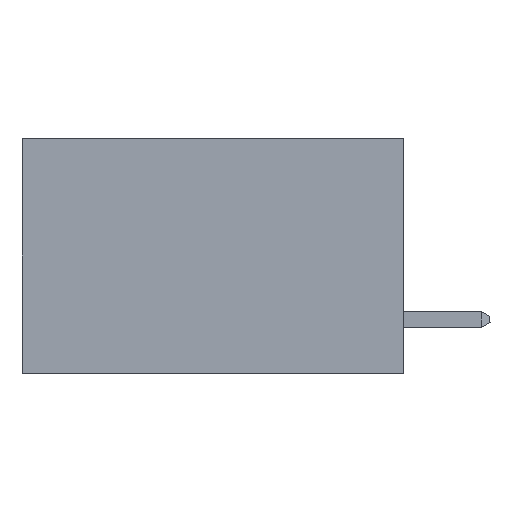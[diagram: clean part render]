
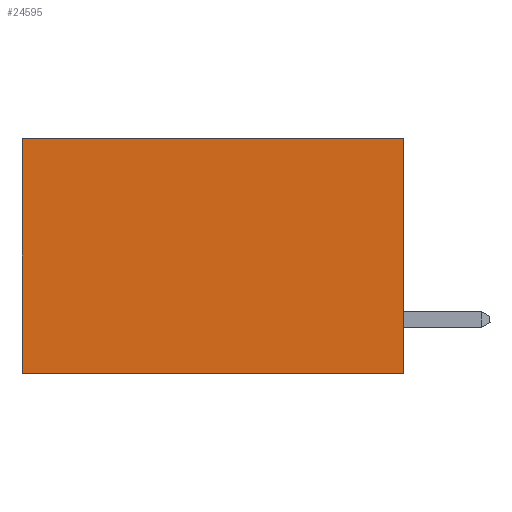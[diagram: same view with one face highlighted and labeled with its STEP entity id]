
A CAD part, left-side view. The second image highlights one B-rep face of the part: STEP entity #24595.
In plain terms, the highlighted planar face has unit normal (-1, 0, 0).
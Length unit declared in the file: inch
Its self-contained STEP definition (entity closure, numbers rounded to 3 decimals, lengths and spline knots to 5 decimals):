
#133 = ORIENTED_EDGE ( 'NONE', *, *, #6053, .F. ) ;
#842 = CARTESIAN_POINT ( 'NONE',  ( 0.2875, 0.6, 0. ) ) ;
#1766 = EDGE_LOOP ( 'NONE', ( #18951, #10182, #133, #32481 ) ) ;
#2347 = AXIS2_PLACEMENT_3D ( 'NONE', #10885, #22368, #5000 ) ;
#3352 = LINE ( 'NONE', #7746, #18024 ) ;
#3517 = CARTESIAN_POINT ( 'NONE',  ( 0.2875, 0., 0. ) ) ;
#3577 = CARTESIAN_POINT ( 'NONE',  ( 0.2875, 0., -0.37 ) ) ;
#5000 = DIRECTION ( 'NONE',  ( 0., 0., -1. ) ) ;
#6053 = EDGE_CURVE ( 'NONE', #13426, #7512, #34824, .T. ) ;
#7512 = VERTEX_POINT ( 'NONE', #3577 ) ;
#7746 = CARTESIAN_POINT ( 'NONE',  ( 0.2875, 0., -0.37 ) ) ;
#8296 = CARTESIAN_POINT ( 'NONE',  ( 0.2875, 0., 0. ) ) ;
#8303 = EDGE_CURVE ( 'NONE', #13763, #11509, #19114, .T. ) ;
#8940 = CARTESIAN_POINT ( 'NONE',  ( 0.2875, 0.6, 0. ) ) ;
#9580 = DIRECTION ( 'NONE',  ( 0., 1., 0. ) ) ;
#10182 = ORIENTED_EDGE ( 'NONE', *, *, #18704, .F. ) ;
#10715 = DIRECTION ( 'NONE',  ( 0., 1., 0. ) ) ;
#10885 = CARTESIAN_POINT ( 'NONE',  ( 0.2875, 0., 0. ) ) ;
#11509 = VERTEX_POINT ( 'NONE', #13775 ) ;
#11645 = CARTESIAN_POINT ( 'NONE',  ( 0.2875, 0., 0. ) ) ;
#13426 = VERTEX_POINT ( 'NONE', #8296 ) ;
#13701 = EDGE_CURVE ( 'NONE', #13426, #13763, #28939, .T. ) ;
#13763 = VERTEX_POINT ( 'NONE', #842 ) ;
#13775 = CARTESIAN_POINT ( 'NONE',  ( 0.2875, 0.6, -0.37 ) ) ;
#18024 = VECTOR ( 'NONE', #10715, 39.37008 ) ;
#18704 = EDGE_CURVE ( 'NONE', #7512, #11509, #3352, .T. ) ;
#18951 = ORIENTED_EDGE ( 'NONE', *, *, #8303, .T. ) ;
#19114 = LINE ( 'NONE', #8940, #25795 ) ;
#19523 = PLANE ( 'NONE',  #2347 ) ;
#19675 = VECTOR ( 'NONE', #37185, 39.37008 ) ;
#22368 = DIRECTION ( 'NONE',  ( 1., 0., 0. ) ) ;
#24595 = ADVANCED_FACE ( 'NONE', ( #29223 ), #19523, .F. ) ;
#25795 = VECTOR ( 'NONE', #31814, 39.37008 ) ;
#28049 = VECTOR ( 'NONE', #9580, 39.37008 ) ;
#28939 = LINE ( 'NONE', #3517, #28049 ) ;
#29223 = FACE_OUTER_BOUND ( 'NONE', #1766, .T. ) ;
#31814 = DIRECTION ( 'NONE',  ( 0., 0., -1. ) ) ;
#32481 = ORIENTED_EDGE ( 'NONE', *, *, #13701, .T. ) ;
#34824 = LINE ( 'NONE', #11645, #19675 ) ;
#37185 = DIRECTION ( 'NONE',  ( 0., 0., -1. ) ) ;
